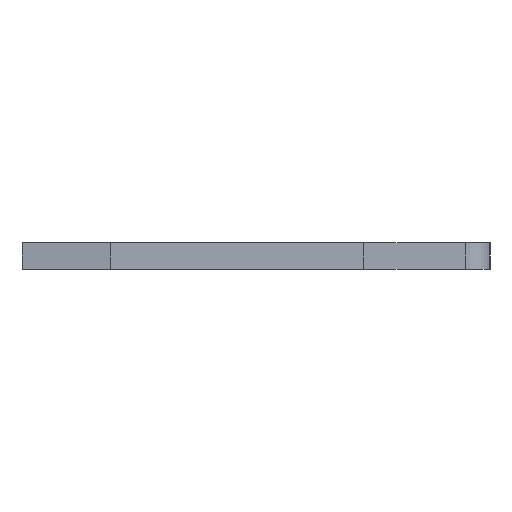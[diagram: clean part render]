
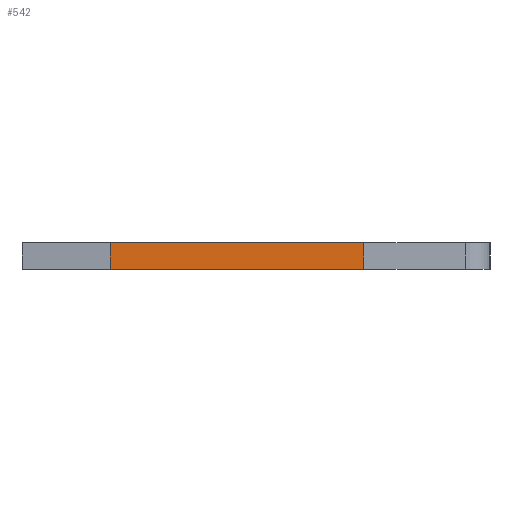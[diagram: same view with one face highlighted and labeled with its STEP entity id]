
A CAD part, left-side view. The second image highlights one B-rep face of the part: STEP entity #542.
In plain terms, the highlighted face is planar.
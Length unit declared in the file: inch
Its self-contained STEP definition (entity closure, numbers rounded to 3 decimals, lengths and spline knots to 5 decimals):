
#59 = LINE ( 'NONE', #1026, #1620 ) ;
#92 = DIRECTION ( 'NONE',  ( -1., 0., 0. ) ) ;
#104 = VERTEX_POINT ( 'NONE', #1592 ) ;
#190 = DIRECTION ( 'NONE',  ( 0., 1., 0. ) ) ;
#199 = ORIENTED_EDGE ( 'NONE', *, *, #381, .T. ) ;
#212 = VERTEX_POINT ( 'NONE', #792 ) ;
#269 = FACE_OUTER_BOUND ( 'NONE', #1959, .T. ) ;
#381 = EDGE_CURVE ( 'NONE', #104, #1110, #709, .T. ) ;
#390 = DIRECTION ( 'NONE',  ( 0., 0., 1. ) ) ;
#542 = ADVANCED_FACE ( 'NONE', ( #269 ), #1787, .F. ) ;
#674 = CARTESIAN_POINT ( 'NONE',  ( -0.013, 0.146, -0.0575 ) ) ;
#682 = EDGE_CURVE ( 'NONE', #714, #104, #59, .T. ) ;
#698 = LINE ( 'NONE', #958, #1516 ) ;
#709 = LINE ( 'NONE', #674, #1329 ) ;
#714 = VERTEX_POINT ( 'NONE', #1644 ) ;
#748 = ORIENTED_EDGE ( 'NONE', *, *, #682, .T. ) ;
#792 = CARTESIAN_POINT ( 'NONE',  ( 0.013, 0.146, -0.0575 ) ) ;
#817 = CARTESIAN_POINT ( 'NONE',  ( -0.013, 0.146, -0.0575 ) ) ;
#854 = DIRECTION ( 'NONE',  ( 1., 0., 0. ) ) ;
#958 = CARTESIAN_POINT ( 'NONE',  ( 0.013, 0.146, -0.0575 ) ) ;
#1003 = CARTESIAN_POINT ( 'NONE',  ( 0.013, 0.146, -0.0575 ) ) ;
#1026 = CARTESIAN_POINT ( 'NONE',  ( 0.013, -0.099, -0.0575 ) ) ;
#1110 = VERTEX_POINT ( 'NONE', #817 ) ;
#1138 = DIRECTION ( 'NONE',  ( -1., 0., 0. ) ) ;
#1142 = DIRECTION ( 'NONE',  ( 0., 1., 0. ) ) ;
#1238 = AXIS2_PLACEMENT_3D ( 'NONE', #1003, #390, #854 ) ;
#1299 = EDGE_CURVE ( 'NONE', #212, #1110, #698, .T. ) ;
#1316 = EDGE_CURVE ( 'NONE', #714, #212, #1848, .T. ) ;
#1329 = VECTOR ( 'NONE', #1142, 39.37008 ) ;
#1351 = VECTOR ( 'NONE', #190, 39.37008 ) ;
#1516 = VECTOR ( 'NONE', #1138, 39.37008 ) ;
#1573 = CARTESIAN_POINT ( 'NONE',  ( 0.013, 0.146, -0.0575 ) ) ;
#1592 = CARTESIAN_POINT ( 'NONE',  ( -0.013, -0.099, -0.0575 ) ) ;
#1620 = VECTOR ( 'NONE', #92, 39.37008 ) ;
#1644 = CARTESIAN_POINT ( 'NONE',  ( 0.013, -0.099, -0.0575 ) ) ;
#1733 = ORIENTED_EDGE ( 'NONE', *, *, #1316, .F. ) ;
#1787 = PLANE ( 'NONE',  #1238 ) ;
#1848 = LINE ( 'NONE', #1573, #1351 ) ;
#1959 = EDGE_LOOP ( 'NONE', ( #199, #1995, #1733, #748 ) ) ;
#1995 = ORIENTED_EDGE ( 'NONE', *, *, #1299, .F. ) ;
